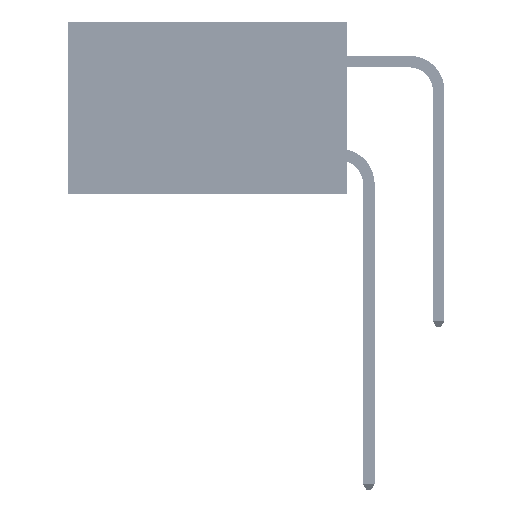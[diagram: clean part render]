
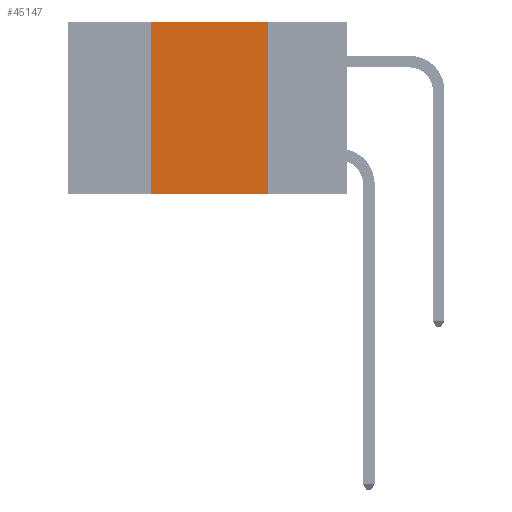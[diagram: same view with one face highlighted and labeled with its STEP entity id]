
A CAD part, left-side view. The second image highlights one B-rep face of the part: STEP entity #45147.
In plain terms, the highlighted planar face has unit normal (-1, 0, 0).
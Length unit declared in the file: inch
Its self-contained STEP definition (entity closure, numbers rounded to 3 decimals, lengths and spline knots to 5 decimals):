
#480 = ORIENTED_EDGE ( 'NONE', *, *, #34184, .T. ) ;
#523 = ORIENTED_EDGE ( 'NONE', *, *, #49477, .F. ) ;
#1922 = VERTEX_POINT ( 'NONE', #48404 ) ;
#5164 = CARTESIAN_POINT ( 'NONE',  ( 0., 0.6, -0.37 ) ) ;
#5234 = AXIS2_PLACEMENT_3D ( 'NONE', #44680, #14245, #44152 ) ;
#8346 = ORIENTED_EDGE ( 'NONE', *, *, #9201, .F. ) ;
#8512 = EDGE_CURVE ( 'NONE', #24616, #1922, #48539, .T. ) ;
#9201 = EDGE_CURVE ( 'NONE', #30434, #24616, #18513, .T. ) ;
#12935 = CARTESIAN_POINT ( 'NONE',  ( 0., 0.17, 0. ) ) ;
#13319 = CARTESIAN_POINT ( 'NONE',  ( 0., 0.42, -0.37 ) ) ;
#14245 = DIRECTION ( 'NONE',  ( 1., 0., 0. ) ) ;
#15964 = ORIENTED_EDGE ( 'NONE', *, *, #8512, .F. ) ;
#17285 = PLANE ( 'NONE',  #5234 ) ;
#18513 = LINE ( 'NONE', #44272, #29950 ) ;
#19570 = VECTOR ( 'NONE', #31744, 39.37008 ) ;
#21120 = LINE ( 'NONE', #49620, #22940 ) ;
#22813 = CARTESIAN_POINT ( 'NONE',  ( 0., 0.17, 0. ) ) ;
#22940 = VECTOR ( 'NONE', #23595, 39.37008 ) ;
#23595 = DIRECTION ( 'NONE',  ( 0., 0., 1. ) ) ;
#24528 = DIRECTION ( 'NONE',  ( 0., 0., -1. ) ) ;
#24616 = VERTEX_POINT ( 'NONE', #22813 ) ;
#26826 = FACE_OUTER_BOUND ( 'NONE', #28272, .T. ) ;
#26879 = CARTESIAN_POINT ( 'NONE',  ( 0., 0.42, 0. ) ) ;
#28272 = EDGE_LOOP ( 'NONE', ( #15964, #8346, #523, #480 ) ) ;
#29795 = LINE ( 'NONE', #5164, #19570 ) ;
#29950 = VECTOR ( 'NONE', #48143, 39.37008 ) ;
#30434 = VERTEX_POINT ( 'NONE', #26879 ) ;
#31744 = DIRECTION ( 'NONE',  ( 0., -1., 0. ) ) ;
#34184 = EDGE_CURVE ( 'NONE', #34842, #1922, #29795, .T. ) ;
#34842 = VERTEX_POINT ( 'NONE', #13319 ) ;
#44152 = DIRECTION ( 'NONE',  ( 0., 0., -1. ) ) ;
#44272 = CARTESIAN_POINT ( 'NONE',  ( 0., 0.6, 0. ) ) ;
#44680 = CARTESIAN_POINT ( 'NONE',  ( 0., 0.6, 0. ) ) ;
#45147 = ADVANCED_FACE ( 'NONE', ( #26826 ), #17285, .F. ) ;
#47964 = VECTOR ( 'NONE', #24528, 39.37008 ) ;
#48143 = DIRECTION ( 'NONE',  ( 0., -1., 0. ) ) ;
#48404 = CARTESIAN_POINT ( 'NONE',  ( 0., 0.17, -0.37 ) ) ;
#48539 = LINE ( 'NONE', #12935, #47964 ) ;
#49477 = EDGE_CURVE ( 'NONE', #34842, #30434, #21120, .T. ) ;
#49620 = CARTESIAN_POINT ( 'NONE',  ( 0., 0.42, 0. ) ) ;
